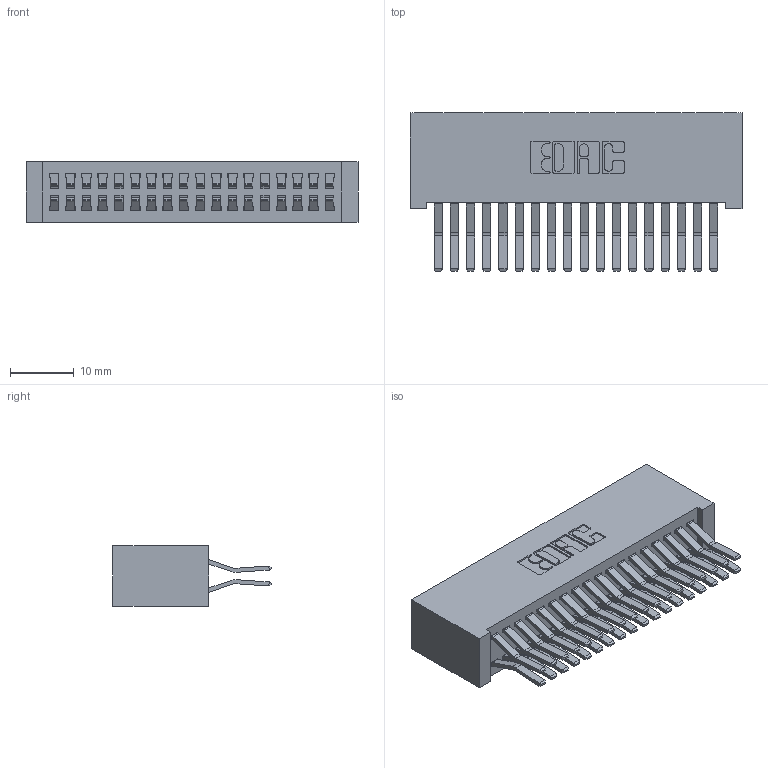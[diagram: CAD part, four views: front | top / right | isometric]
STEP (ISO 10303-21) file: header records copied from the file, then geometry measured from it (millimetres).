
FILE_DESCRIPTION (( 'STEP AP203' ), '1' );
FILE_NAME ('392-036-560-201.STEP', '2018-08-16T04:05:34', ( '' ), ( '' ), 'SwSTEP 2.0', 'SolidWorks 2016', '' );
FILE_SCHEMA (( 'CONFIG_CONTROL_DESIGN' ));
Length unit declared in the file: inch
Products named in the file (3): 345-292-001_560 Tail; 392-036-560-201; 342 Part_Lugless
Assembly tree (37 placements, depth 2):
  392-036-560-201
    342 Part_Lugless
    345-292-001_560 Tail  x36
Bounding box: 51.97 x 24.78 x 9.4 mm (x, y, z)
Volume: 5231.6 mm3; surface area: 8937.4 mm2
Topology: 37 solids, 37 shells, 2046 faces, 6071 edges, 3998 vertices
Faces by surface type: plane 1358, cylinder 688
Entity records: 14363 total; most frequent: CARTESIAN_POINT 2406, ORIENTED_EDGE 2342, DIRECTION 2095, EDGE_CURVE 1171, VECTOR 1047, LINE 1047, VERTEX_POINT 778, AXIS2_PLACEMENT_3D 524
